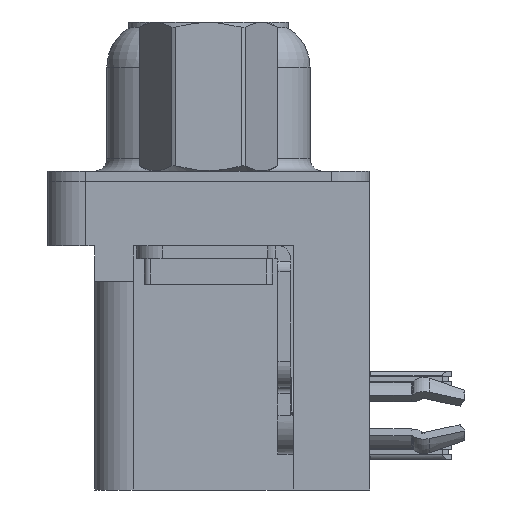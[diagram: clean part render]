
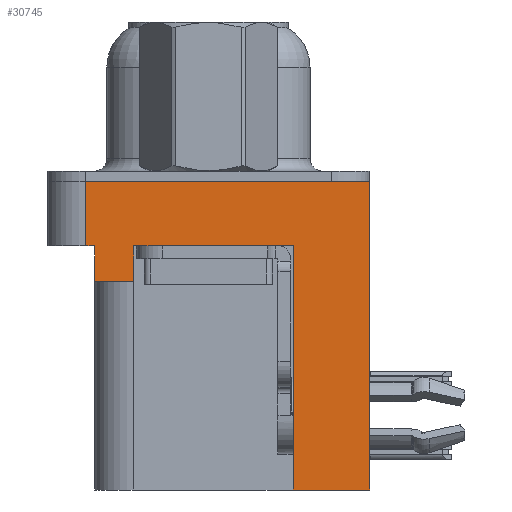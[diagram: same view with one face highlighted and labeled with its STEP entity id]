
A CAD part, left-side view. The second image highlights one B-rep face of the part: STEP entity #30745.
In plain terms, the highlighted planar face has unit normal (-1, 0, 0).
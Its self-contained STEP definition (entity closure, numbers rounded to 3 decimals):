
#183 = LINE ( 'NONE', #4687, #28583 ) ;
#765 = CARTESIAN_POINT ( 'NONE',  ( -3., -6.275, -2.5 ) ) ;
#1006 = CARTESIAN_POINT ( 'NONE',  ( -3., -6.275, 0. ) ) ;
#1963 = CARTESIAN_POINT ( 'NONE',  ( -3., 4.425, -2.5 ) ) ;
#2712 = CARTESIAN_POINT ( 'NONE',  ( -3., -3.295, -2.5 ) ) ;
#4482 = ORIENTED_EDGE ( 'NONE', *, *, #29281, .F. ) ;
#4523 = VECTOR ( 'NONE', #19334, 1000. ) ;
#4687 = CARTESIAN_POINT ( 'NONE',  ( -3., -3.295, -12. ) ) ;
#5170 = LINE ( 'NONE', #22568, #11054 ) ;
#5999 = CARTESIAN_POINT ( 'NONE',  ( -3., 4.425, -3.9 ) ) ;
#6356 = CARTESIAN_POINT ( 'NONE',  ( -3., 2.895, -2.5 ) ) ;
#6495 = CARTESIAN_POINT ( 'NONE',  ( -3., 2.895, -3.9 ) ) ;
#8865 = VECTOR ( 'NONE', #28523, 1000. ) ;
#8875 = EDGE_CURVE ( 'NONE', #19816, #35753, #11541, .T. ) ;
#9638 = CARTESIAN_POINT ( 'NONE',  ( -3., -3.295, -12. ) ) ;
#9767 = ORIENTED_EDGE ( 'NONE', *, *, #17792, .F. ) ;
#10526 = EDGE_CURVE ( 'NONE', #28563, #19816, #28019, .T. ) ;
#11054 = VECTOR ( 'NONE', #11364, 1000. ) ;
#11193 = VERTEX_POINT ( 'NONE', #1963 ) ;
#11245 = LINE ( 'NONE', #36304, #12137 ) ;
#11364 = DIRECTION ( 'NONE',  ( 0., 0., 1. ) ) ;
#11541 = LINE ( 'NONE', #765, #37207 ) ;
#11550 = DIRECTION ( 'NONE',  ( 0., 0., 1. ) ) ;
#11794 = DIRECTION ( 'NONE',  ( 0., 0., 1. ) ) ;
#12137 = VECTOR ( 'NONE', #19067, 1000. ) ;
#12345 = LINE ( 'NONE', #9638, #19115 ) ;
#13048 = ORIENTED_EDGE ( 'NONE', *, *, #26241, .F. ) ;
#13194 = VECTOR ( 'NONE', #11550, 1000. ) ;
#13809 = CARTESIAN_POINT ( 'NONE',  ( -3., -6.275, -2.5 ) ) ;
#14235 = ORIENTED_EDGE ( 'NONE', *, *, #8875, .T. ) ;
#14254 = CARTESIAN_POINT ( 'NONE',  ( -3., 4.775, -2.5 ) ) ;
#14452 = DIRECTION ( 'NONE',  ( -1., 0., 0. ) ) ;
#14944 = VECTOR ( 'NONE', #15671, 1000. ) ;
#15671 = DIRECTION ( 'NONE',  ( 0., -1., 0. ) ) ;
#15970 = VERTEX_POINT ( 'NONE', #25523 ) ;
#16593 = ORIENTED_EDGE ( 'NONE', *, *, #10526, .T. ) ;
#16799 = CARTESIAN_POINT ( 'NONE',  ( -3., 4.425, -3.9 ) ) ;
#17315 = ORIENTED_EDGE ( 'NONE', *, *, #23055, .F. ) ;
#17344 = CARTESIAN_POINT ( 'NONE',  ( -3., -3.295, -12. ) ) ;
#17792 = EDGE_CURVE ( 'NONE', #18032, #24351, #23297, .T. ) ;
#17999 = ORIENTED_EDGE ( 'NONE', *, *, #20471, .T. ) ;
#18032 = VERTEX_POINT ( 'NONE', #30777 ) ;
#18557 = LINE ( 'NONE', #1006, #14944 ) ;
#18833 = EDGE_CURVE ( 'NONE', #28563, #36382, #32246, .T. ) ;
#19067 = DIRECTION ( 'NONE',  ( 0., 0., 1. ) ) ;
#19115 = VECTOR ( 'NONE', #20836, 1000. ) ;
#19334 = DIRECTION ( 'NONE',  ( 0., -1., 0. ) ) ;
#19776 = VERTEX_POINT ( 'NONE', #17344 ) ;
#19816 = VERTEX_POINT ( 'NONE', #6356 ) ;
#20120 = ORIENTED_EDGE ( 'NONE', *, *, #24415, .F. ) ;
#20471 = EDGE_CURVE ( 'NONE', #21187, #15970, #5170, .T. ) ;
#20836 = DIRECTION ( 'NONE',  ( 0., 0., 1. ) ) ;
#21187 = VERTEX_POINT ( 'NONE', #31531 ) ;
#22568 = CARTESIAN_POINT ( 'NONE',  ( -3., -6.275, -2.5 ) ) ;
#23055 = EDGE_CURVE ( 'NONE', #24351, #15970, #18557, .T. ) ;
#23297 = LINE ( 'NONE', #14254, #8865 ) ;
#24351 = VERTEX_POINT ( 'NONE', #24723 ) ;
#24415 = EDGE_CURVE ( 'NONE', #36382, #11193, #11245, .T. ) ;
#24723 = CARTESIAN_POINT ( 'NONE',  ( -3., 4.775, 0. ) ) ;
#25523 = CARTESIAN_POINT ( 'NONE',  ( -3., -6.275, 0. ) ) ;
#25812 = CARTESIAN_POINT ( 'NONE',  ( -3., 2.895, -3.9 ) ) ;
#26216 = DIRECTION ( 'NONE',  ( 0., 1., 0. ) ) ;
#26241 = EDGE_CURVE ( 'NONE', #19776, #35753, #12345, .T. ) ;
#26517 = EDGE_LOOP ( 'NONE', ( #17315, #9767, #35736, #20120, #35305, #16593, #14235, #13048, #4482, #17999 ) ) ;
#28019 = LINE ( 'NONE', #6495, #13194 ) ;
#28523 = DIRECTION ( 'NONE',  ( 0., 0., 1. ) ) ;
#28563 = VERTEX_POINT ( 'NONE', #25812 ) ;
#28583 = VECTOR ( 'NONE', #30459, 1000. ) ;
#28723 = CARTESIAN_POINT ( 'NONE',  ( -3., -6.275, -2.5 ) ) ;
#29281 = EDGE_CURVE ( 'NONE', #21187, #19776, #183, .T. ) ;
#29605 = DIRECTION ( 'NONE',  ( 0., -1., 0. ) ) ;
#30459 = DIRECTION ( 'NONE',  ( 0., 1., 0. ) ) ;
#30478 = VECTOR ( 'NONE', #26216, 1000. ) ;
#30617 = LINE ( 'NONE', #13809, #4523 ) ;
#30745 = ADVANCED_FACE ( 'NONE', ( #31684 ), #34219, .T. ) ;
#30777 = CARTESIAN_POINT ( 'NONE',  ( -3., 4.775, -2.5 ) ) ;
#31314 = AXIS2_PLACEMENT_3D ( 'NONE', #28723, #14452, #11794 ) ;
#31531 = CARTESIAN_POINT ( 'NONE',  ( -3., -6.275, -12. ) ) ;
#31684 = FACE_OUTER_BOUND ( 'NONE', #26517, .T. ) ;
#32246 = LINE ( 'NONE', #5999, #30478 ) ;
#33537 = EDGE_CURVE ( 'NONE', #18032, #11193, #30617, .T. ) ;
#34219 = PLANE ( 'NONE',  #31314 ) ;
#35305 = ORIENTED_EDGE ( 'NONE', *, *, #18833, .F. ) ;
#35736 = ORIENTED_EDGE ( 'NONE', *, *, #33537, .T. ) ;
#35753 = VERTEX_POINT ( 'NONE', #2712 ) ;
#36304 = CARTESIAN_POINT ( 'NONE',  ( -3., 4.425, -3.9 ) ) ;
#36382 = VERTEX_POINT ( 'NONE', #16799 ) ;
#37207 = VECTOR ( 'NONE', #29605, 1000. ) ;
